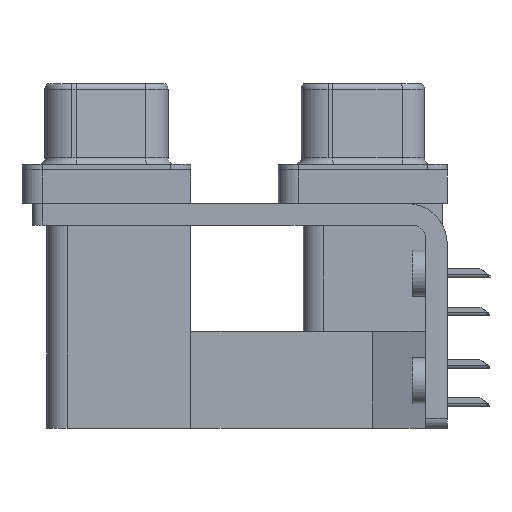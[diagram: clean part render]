
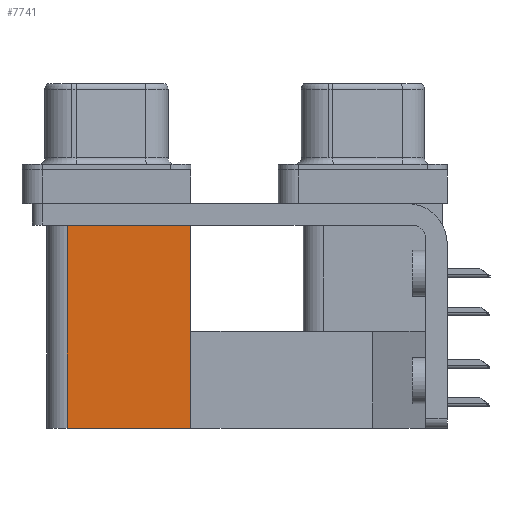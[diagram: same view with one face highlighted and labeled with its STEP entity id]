
A CAD part, left-side view. The second image highlights one B-rep face of the part: STEP entity #7741.
In plain terms, the highlighted planar face has unit normal (-1, 0, 0).
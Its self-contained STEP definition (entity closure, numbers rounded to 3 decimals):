
#73 = DIRECTION ( 'NONE',  ( 0., 1., 0. ) ) ;
#578 = DIRECTION ( 'NONE',  ( 1., 0., 0. ) ) ;
#2733 = AXIS2_PLACEMENT_3D ( 'NONE', #26578, #578, #26709 ) ;
#3694 = VERTEX_POINT ( 'NONE', #18109 ) ;
#4572 = LINE ( 'NONE', #23874, #15722 ) ;
#5558 = VECTOR ( 'NONE', #8850, 1000. ) ;
#5744 = ORIENTED_EDGE ( 'NONE', *, *, #16796, .F. ) ;
#6263 = CARTESIAN_POINT ( 'NONE',  ( 3.79, 12.775, -2.5 ) ) ;
#6715 = DIRECTION ( 'NONE',  ( 0., 0., 1. ) ) ;
#7052 = VERTEX_POINT ( 'NONE', #26046 ) ;
#7741 = ADVANCED_FACE ( 'NONE', ( #9148 ), #17860, .F. ) ;
#7777 = VERTEX_POINT ( 'NONE', #21265 ) ;
#8274 = EDGE_CURVE ( 'NONE', #7052, #3694, #8624, .T. ) ;
#8624 = LINE ( 'NONE', #21788, #11878 ) ;
#8850 = DIRECTION ( 'NONE',  ( 0., 1., 0. ) ) ;
#9148 = FACE_OUTER_BOUND ( 'NONE', #27325, .T. ) ;
#9297 = VERTEX_POINT ( 'NONE', #12739 ) ;
#10527 = ORIENTED_EDGE ( 'NONE', *, *, #13663, .T. ) ;
#11878 = VECTOR ( 'NONE', #73, 1000. ) ;
#12739 = CARTESIAN_POINT ( 'NONE',  ( 3.79, 12.775, -2.5 ) ) ;
#13663 = EDGE_CURVE ( 'NONE', #7052, #9297, #4572, .T. ) ;
#15722 = VECTOR ( 'NONE', #6715, 1000. ) ;
#16796 = EDGE_CURVE ( 'NONE', #3694, #7777, #17877, .T. ) ;
#17860 = PLANE ( 'NONE',  #2733 ) ;
#17877 = LINE ( 'NONE', #26857, #25203 ) ;
#18109 = CARTESIAN_POINT ( 'NONE',  ( 3.79, 21.975, -19.2 ) ) ;
#18572 = EDGE_CURVE ( 'NONE', #9297, #7777, #26151, .T. ) ;
#21265 = CARTESIAN_POINT ( 'NONE',  ( 3.79, 21.975, -2.5 ) ) ;
#21788 = CARTESIAN_POINT ( 'NONE',  ( 3.79, 12.775, -19.2 ) ) ;
#23874 = CARTESIAN_POINT ( 'NONE',  ( 3.79, 12.775, -19.2 ) ) ;
#24578 = DIRECTION ( 'NONE',  ( 0., 0., 1. ) ) ;
#25203 = VECTOR ( 'NONE', #24578, 1000. ) ;
#25632 = ORIENTED_EDGE ( 'NONE', *, *, #8274, .F. ) ;
#26046 = CARTESIAN_POINT ( 'NONE',  ( 3.79, 12.775, -19.2 ) ) ;
#26133 = ORIENTED_EDGE ( 'NONE', *, *, #18572, .T. ) ;
#26151 = LINE ( 'NONE', #6263, #5558 ) ;
#26578 = CARTESIAN_POINT ( 'NONE',  ( 3.79, 12.775, -19.2 ) ) ;
#26709 = DIRECTION ( 'NONE',  ( 0., 1., 0. ) ) ;
#26857 = CARTESIAN_POINT ( 'NONE',  ( 3.79, 21.975, -19.2 ) ) ;
#27325 = EDGE_LOOP ( 'NONE', ( #26133, #5744, #25632, #10527 ) ) ;
